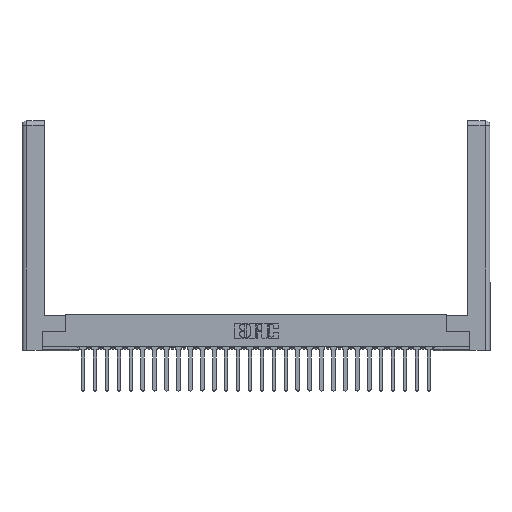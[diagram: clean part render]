
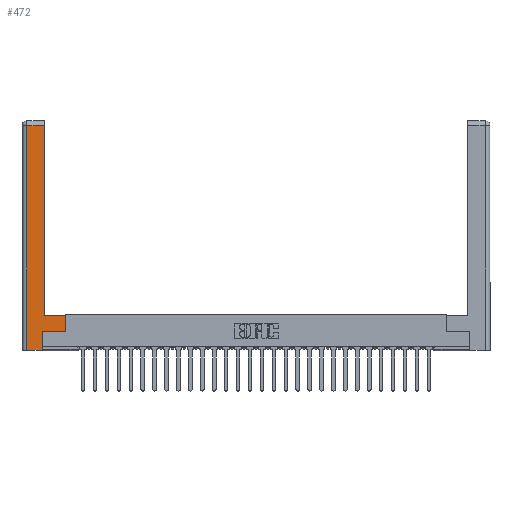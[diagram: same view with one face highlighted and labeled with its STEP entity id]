
A CAD part, top view. The second image highlights one B-rep face of the part: STEP entity #472.
In plain terms, the highlighted planar face has unit normal (0, 0, 1).
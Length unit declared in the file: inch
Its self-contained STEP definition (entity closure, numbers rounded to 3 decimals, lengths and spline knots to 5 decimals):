
#14 = ORIENTED_EDGE ( 'NONE', *, *, #25348, .T. ) ;
#128 = VECTOR ( 'NONE', #3788, 39.37008 ) ;
#472 = ADVANCED_FACE ( 'NONE', ( #4897 ), #26700, .F. ) ;
#834 = VECTOR ( 'NONE', #19518, 39.37008 ) ;
#1205 = VECTOR ( 'NONE', #21411, 39.37008 ) ;
#1241 = LINE ( 'NONE', #5255, #1205 ) ;
#1442 = EDGE_CURVE ( 'NONE', #3683, #2638, #24305, .T. ) ;
#1446 = CARTESIAN_POINT ( 'NONE',  ( 0.265, 0.245, 0. ) ) ;
#2638 = VERTEX_POINT ( 'NONE', #2657 ) ;
#2657 = CARTESIAN_POINT ( 'NONE',  ( 0.295, 0.45, 0. ) ) ;
#2975 = ORIENTED_EDGE ( 'NONE', *, *, #19223, .T. ) ;
#3673 = CARTESIAN_POINT ( 'NONE',  ( 0.0615, 2.94, 0. ) ) ;
#3683 = VERTEX_POINT ( 'NONE', #19195 ) ;
#3788 = DIRECTION ( 'NONE',  ( 1., 0., 0. ) ) ;
#4897 = FACE_OUTER_BOUND ( 'NONE', #24411, .T. ) ;
#5255 = CARTESIAN_POINT ( 'NONE',  ( 0.295, 3., 0. ) ) ;
#6010 = CARTESIAN_POINT ( 'NONE',  ( 0.0615, 2.94, 0. ) ) ;
#6823 = CARTESIAN_POINT ( 'NONE',  ( 0.265, 0., 0. ) ) ;
#8493 = CARTESIAN_POINT ( 'NONE',  ( 0., 0., 0. ) ) ;
#8712 = VECTOR ( 'NONE', #13583, 39.37008 ) ;
#8733 = ORIENTED_EDGE ( 'NONE', *, *, #12637, .T. ) ;
#8956 = DIRECTION ( 'NONE',  ( -1., 0., 0. ) ) ;
#9371 = DIRECTION ( 'NONE',  ( 0., 0., -1. ) ) ;
#9773 = EDGE_CURVE ( 'NONE', #14873, #12012, #18988, .T. ) ;
#10243 = VECTOR ( 'NONE', #8956, 39.37008 ) ;
#10573 = CARTESIAN_POINT ( 'NONE',  ( 0.565, 0.45, 0. ) ) ;
#10867 = CARTESIAN_POINT ( 'NONE',  ( 0.295, 0.45, 0. ) ) ;
#12012 = VERTEX_POINT ( 'NONE', #6010 ) ;
#12052 = CARTESIAN_POINT ( 'NONE',  ( 0.265, 0.245, 0. ) ) ;
#12637 = EDGE_CURVE ( 'NONE', #25721, #3683, #25684, .T. ) ;
#13516 = CARTESIAN_POINT ( 'NONE',  ( 0.0615, 0., 0. ) ) ;
#13583 = DIRECTION ( 'NONE',  ( 1., 0., 0. ) ) ;
#13698 = EDGE_CURVE ( 'NONE', #22287, #25721, #19078, .T. ) ;
#14275 = DIRECTION ( 'NONE',  ( -1., 0., 0. ) ) ;
#14873 = VERTEX_POINT ( 'NONE', #22689 ) ;
#15513 = DIRECTION ( 'NONE',  ( -1., 0., 0. ) ) ;
#18054 = ORIENTED_EDGE ( 'NONE', *, *, #24833, .T. ) ;
#18948 = ORIENTED_EDGE ( 'NONE', *, *, #13698, .T. ) ;
#18988 = LINE ( 'NONE', #3673, #24814 ) ;
#19078 = LINE ( 'NONE', #22467, #8712 ) ;
#19195 = CARTESIAN_POINT ( 'NONE',  ( 0.565, 0.45, 0. ) ) ;
#19223 = EDGE_CURVE ( 'NONE', #12012, #28729, #27992, .T. ) ;
#19518 = DIRECTION ( 'NONE',  ( 0., 1., 0. ) ) ;
#20138 = AXIS2_PLACEMENT_3D ( 'NONE', #8493, #9371, #14275 ) ;
#20627 = CARTESIAN_POINT ( 'NONE',  ( 0.0615, 0., 0. ) ) ;
#20849 = CARTESIAN_POINT ( 'NONE',  ( 0.565, 0.245, 0. ) ) ;
#21083 = DIRECTION ( 'NONE',  ( 0., 1., 0. ) ) ;
#21411 = DIRECTION ( 'NONE',  ( 0., 1., 0. ) ) ;
#21876 = VECTOR ( 'NONE', #29821, 39.37008 ) ;
#22287 = VERTEX_POINT ( 'NONE', #1446 ) ;
#22467 = CARTESIAN_POINT ( 'NONE',  ( 0.565, 0.245, 0. ) ) ;
#22689 = CARTESIAN_POINT ( 'NONE',  ( 0.295, 2.94, 0. ) ) ;
#22843 = EDGE_CURVE ( 'NONE', #28421, #22287, #23669, .T. ) ;
#23297 = VECTOR ( 'NONE', #21083, 39.37008 ) ;
#23669 = LINE ( 'NONE', #12052, #23297 ) ;
#24300 = ORIENTED_EDGE ( 'NONE', *, *, #22843, .T. ) ;
#24305 = LINE ( 'NONE', #10867, #10243 ) ;
#24411 = EDGE_LOOP ( 'NONE', ( #14, #24653, #2975, #18054, #24300, #18948, #8733, #24920 ) ) ;
#24653 = ORIENTED_EDGE ( 'NONE', *, *, #9773, .T. ) ;
#24814 = VECTOR ( 'NONE', #15513, 39.37008 ) ;
#24833 = EDGE_CURVE ( 'NONE', #28729, #28421, #29659, .T. ) ;
#24920 = ORIENTED_EDGE ( 'NONE', *, *, #1442, .T. ) ;
#25348 = EDGE_CURVE ( 'NONE', #2638, #14873, #1241, .T. ) ;
#25684 = LINE ( 'NONE', #10573, #834 ) ;
#25721 = VERTEX_POINT ( 'NONE', #20849 ) ;
#26700 = PLANE ( 'NONE',  #20138 ) ;
#27992 = LINE ( 'NONE', #13516, #21876 ) ;
#28386 = CARTESIAN_POINT ( 'NONE',  ( 0.265, 0., 0. ) ) ;
#28421 = VERTEX_POINT ( 'NONE', #6823 ) ;
#28729 = VERTEX_POINT ( 'NONE', #20627 ) ;
#29659 = LINE ( 'NONE', #28386, #128 ) ;
#29821 = DIRECTION ( 'NONE',  ( 0., -1., 0. ) ) ;
